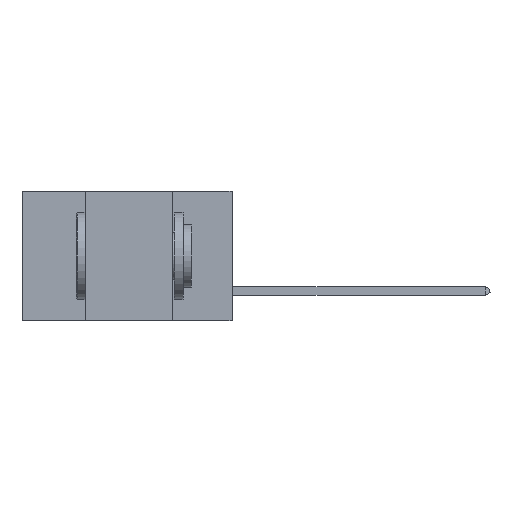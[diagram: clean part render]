
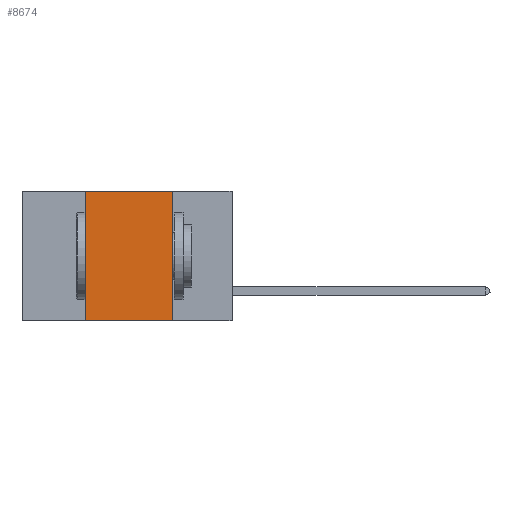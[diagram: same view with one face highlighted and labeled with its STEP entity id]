
A CAD part, left-side view. The second image highlights one B-rep face of the part: STEP entity #8674.
In plain terms, the highlighted planar face has unit normal (-1, 0, 0).
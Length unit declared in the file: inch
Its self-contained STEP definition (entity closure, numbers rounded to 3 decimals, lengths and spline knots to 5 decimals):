
#51 = EDGE_CURVE ( 'NONE', #21385, #14820, #17916, .T. ) ;
#1051 = EDGE_CURVE ( 'NONE', #6368, #26252, #19474, .T. ) ;
#1343 = FACE_OUTER_BOUND ( 'NONE', #31529, .T. ) ;
#1914 = CARTESIAN_POINT ( 'NONE',  ( 0., 0.42, -0.37 ) ) ;
#4519 = CARTESIAN_POINT ( 'NONE',  ( 0., 0.6, 0. ) ) ;
#4712 = DIRECTION ( 'NONE',  ( 0., 0., 1. ) ) ;
#5938 = LINE ( 'NONE', #24321, #15865 ) ;
#6368 = VERTEX_POINT ( 'NONE', #1914 ) ;
#7247 = CARTESIAN_POINT ( 'NONE',  ( 0., 0.6, -0.37 ) ) ;
#7396 = CARTESIAN_POINT ( 'NONE',  ( 0., 0.17, -0.37 ) ) ;
#8594 = DIRECTION ( 'NONE',  ( 1., 0., 0. ) ) ;
#8674 = ADVANCED_FACE ( 'NONE', ( #1343 ), #25802, .F. ) ;
#8862 = CARTESIAN_POINT ( 'NONE',  ( 0., 0.17, 0. ) ) ;
#9809 = DIRECTION ( 'NONE',  ( 0., -1., 0. ) ) ;
#9962 = VECTOR ( 'NONE', #4712, 39.37008 ) ;
#10860 = DIRECTION ( 'NONE',  ( 0., 0., -1. ) ) ;
#11715 = DIRECTION ( 'NONE',  ( 0., -1., 0. ) ) ;
#11898 = ORIENTED_EDGE ( 'NONE', *, *, #1051, .T. ) ;
#12617 = VECTOR ( 'NONE', #9809, 39.37008 ) ;
#13082 = AXIS2_PLACEMENT_3D ( 'NONE', #18191, #8594, #10860 ) ;
#13623 = ORIENTED_EDGE ( 'NONE', *, *, #23794, .F. ) ;
#13633 = ORIENTED_EDGE ( 'NONE', *, *, #30069, .F. ) ;
#14316 = ORIENTED_EDGE ( 'NONE', *, *, #51, .F. ) ;
#14820 = VERTEX_POINT ( 'NONE', #8862 ) ;
#15865 = VECTOR ( 'NONE', #21399, 39.37008 ) ;
#17838 = CARTESIAN_POINT ( 'NONE',  ( 0., 0.42, 0. ) ) ;
#17916 = LINE ( 'NONE', #4519, #27607 ) ;
#18191 = CARTESIAN_POINT ( 'NONE',  ( 0., 0.6, 0. ) ) ;
#19474 = LINE ( 'NONE', #7247, #12617 ) ;
#21385 = VERTEX_POINT ( 'NONE', #17838 ) ;
#21399 = DIRECTION ( 'NONE',  ( 0., 0., -1. ) ) ;
#22048 = CARTESIAN_POINT ( 'NONE',  ( 0., 0.42, 0. ) ) ;
#23794 = EDGE_CURVE ( 'NONE', #6368, #21385, #30311, .T. ) ;
#24321 = CARTESIAN_POINT ( 'NONE',  ( 0., 0.17, 0. ) ) ;
#25802 = PLANE ( 'NONE',  #13082 ) ;
#26252 = VERTEX_POINT ( 'NONE', #7396 ) ;
#27607 = VECTOR ( 'NONE', #11715, 39.37008 ) ;
#30069 = EDGE_CURVE ( 'NONE', #14820, #26252, #5938, .T. ) ;
#30311 = LINE ( 'NONE', #22048, #9962 ) ;
#31529 = EDGE_LOOP ( 'NONE', ( #13633, #14316, #13623, #11898 ) ) ;
